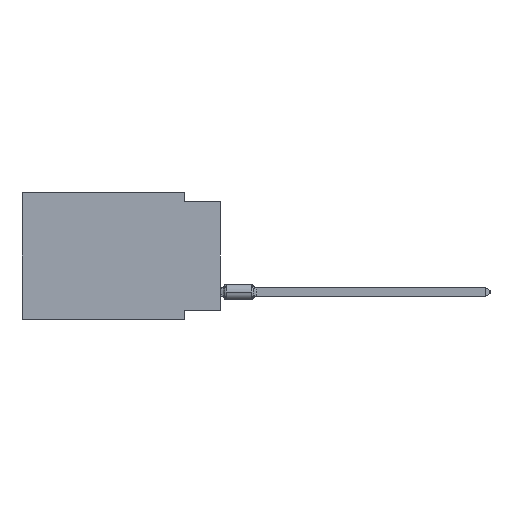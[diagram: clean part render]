
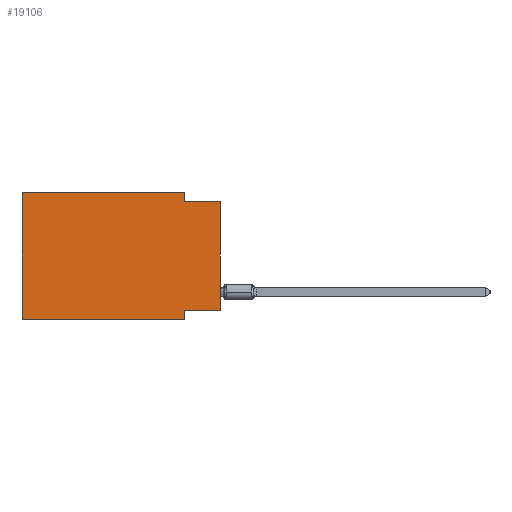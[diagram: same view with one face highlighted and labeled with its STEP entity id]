
A CAD part, left-side view. The second image highlights one B-rep face of the part: STEP entity #19106.
In plain terms, the highlighted planar face has unit normal (-1, 0, 0).
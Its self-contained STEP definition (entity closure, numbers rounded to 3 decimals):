
#842 = EDGE_CURVE ( 'NONE', #40136, #6091, #41778, .T. ) ;
#1027 = DIRECTION ( 'NONE',  ( 0., 1., 0. ) ) ;
#1290 = EDGE_CURVE ( 'NONE', #2727, #6091, #23834, .T. ) ;
#1426 = DIRECTION ( 'NONE',  ( 0., 0., -1. ) ) ;
#1593 = VECTOR ( 'NONE', #2149, 1000. ) ;
#1830 = CARTESIAN_POINT ( 'NONE',  ( 0., 2.54, -8.89 ) ) ;
#2149 = DIRECTION ( 'NONE',  ( 0., 0., 1. ) ) ;
#2727 = VERTEX_POINT ( 'NONE', #15094 ) ;
#3923 = CARTESIAN_POINT ( 'NONE',  ( 0., 13.97, -8.89 ) ) ;
#4851 = DIRECTION ( 'NONE',  ( 0., 0., 1. ) ) ;
#5412 = EDGE_LOOP ( 'NONE', ( #22306, #21346, #14038, #32604, #29461, #24271, #34943, #39849 ) ) ;
#6091 = VERTEX_POINT ( 'NONE', #12568 ) ;
#8406 = VERTEX_POINT ( 'NONE', #26233 ) ;
#8690 = VERTEX_POINT ( 'NONE', #37290 ) ;
#12050 = LINE ( 'NONE', #19591, #24294 ) ;
#12185 = LINE ( 'NONE', #12821, #35570 ) ;
#12255 = CARTESIAN_POINT ( 'NONE',  ( 0., 13.97, 0. ) ) ;
#12556 = VERTEX_POINT ( 'NONE', #3923 ) ;
#12568 = CARTESIAN_POINT ( 'NONE',  ( 0., 0., -0.635 ) ) ;
#12821 = CARTESIAN_POINT ( 'NONE',  ( 0., 2.54, -8.89 ) ) ;
#13367 = VECTOR ( 'NONE', #1426, 1000. ) ;
#13595 = LINE ( 'NONE', #21150, #13966 ) ;
#13966 = VECTOR ( 'NONE', #1027, 1000. ) ;
#14038 = ORIENTED_EDGE ( 'NONE', *, *, #28883, .F. ) ;
#15094 = CARTESIAN_POINT ( 'NONE',  ( 0., 2.54, -0.635 ) ) ;
#15495 = FACE_OUTER_BOUND ( 'NONE', #5412, .T. ) ;
#15940 = VECTOR ( 'NONE', #4851, 1000. ) ;
#16225 = CARTESIAN_POINT ( 'NONE',  ( 0., 13.97, -8.89 ) ) ;
#16342 = DIRECTION ( 'NONE',  ( 0., 0., -1. ) ) ;
#17888 = CARTESIAN_POINT ( 'NONE',  ( 0., 2.54, 0. ) ) ;
#18266 = CARTESIAN_POINT ( 'NONE',  ( 0., 13.97, 0. ) ) ;
#19106 = ADVANCED_FACE ( 'NONE', ( #15495 ), #28709, .F. ) ;
#19591 = CARTESIAN_POINT ( 'NONE',  ( 0., 13.97, 0. ) ) ;
#21131 = EDGE_CURVE ( 'NONE', #40136, #8690, #13595, .T. ) ;
#21150 = CARTESIAN_POINT ( 'NONE',  ( 0., 0., -8.255 ) ) ;
#21346 = ORIENTED_EDGE ( 'NONE', *, *, #1290, .F. ) ;
#22176 = DIRECTION ( 'NONE',  ( 1., 0., 0. ) ) ;
#22306 = ORIENTED_EDGE ( 'NONE', *, *, #842, .T. ) ;
#22615 = DIRECTION ( 'NONE',  ( 0., -1., 0. ) ) ;
#22690 = DIRECTION ( 'NONE',  ( 0., -1., 0. ) ) ;
#23834 = LINE ( 'NONE', #34868, #36885 ) ;
#24271 = ORIENTED_EDGE ( 'NONE', *, *, #41585, .T. ) ;
#24294 = VECTOR ( 'NONE', #22615, 1000. ) ;
#24336 = VERTEX_POINT ( 'NONE', #1830 ) ;
#25329 = DIRECTION ( 'NONE',  ( 0., -1., 0. ) ) ;
#25997 = DIRECTION ( 'NONE',  ( 0., 0., -1. ) ) ;
#26233 = CARTESIAN_POINT ( 'NONE',  ( 0., 2.54, 0. ) ) ;
#28709 = PLANE ( 'NONE',  #30386 ) ;
#28883 = EDGE_CURVE ( 'NONE', #8406, #2727, #30878, .T. ) ;
#29461 = ORIENTED_EDGE ( 'NONE', *, *, #30569, .F. ) ;
#30386 = AXIS2_PLACEMENT_3D ( 'NONE', #12255, #22176, #16342 ) ;
#30569 = EDGE_CURVE ( 'NONE', #12556, #42807, #34713, .T. ) ;
#30878 = LINE ( 'NONE', #17888, #13367 ) ;
#31461 = EDGE_CURVE ( 'NONE', #42807, #8406, #12050, .T. ) ;
#31809 = CARTESIAN_POINT ( 'NONE',  ( 0., 0., 0. ) ) ;
#32604 = ORIENTED_EDGE ( 'NONE', *, *, #31461, .F. ) ;
#34713 = LINE ( 'NONE', #18266, #15940 ) ;
#34868 = CARTESIAN_POINT ( 'NONE',  ( 0., 0., -0.635 ) ) ;
#34943 = ORIENTED_EDGE ( 'NONE', *, *, #35955, .F. ) ;
#35077 = LINE ( 'NONE', #16225, #37457 ) ;
#35570 = VECTOR ( 'NONE', #25997, 1000. ) ;
#35955 = EDGE_CURVE ( 'NONE', #8690, #24336, #12185, .T. ) ;
#36885 = VECTOR ( 'NONE', #25329, 1000. ) ;
#37290 = CARTESIAN_POINT ( 'NONE',  ( 0., 2.54, -8.255 ) ) ;
#37457 = VECTOR ( 'NONE', #22690, 1000. ) ;
#39181 = CARTESIAN_POINT ( 'NONE',  ( 0., 13.97, 0. ) ) ;
#39849 = ORIENTED_EDGE ( 'NONE', *, *, #21131, .F. ) ;
#40136 = VERTEX_POINT ( 'NONE', #42238 ) ;
#41585 = EDGE_CURVE ( 'NONE', #12556, #24336, #35077, .T. ) ;
#41778 = LINE ( 'NONE', #31809, #1593 ) ;
#42238 = CARTESIAN_POINT ( 'NONE',  ( 0., 0., -8.255 ) ) ;
#42807 = VERTEX_POINT ( 'NONE', #39181 ) ;
